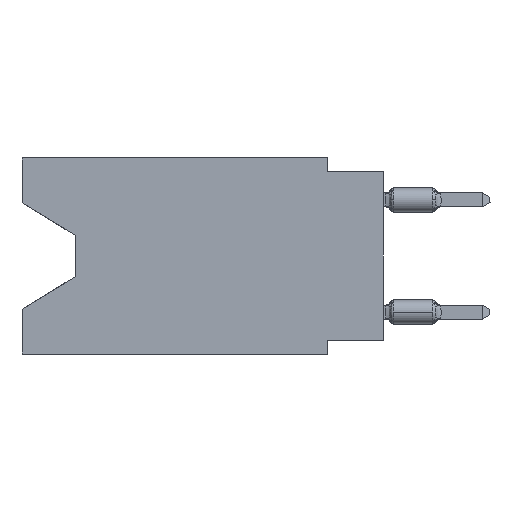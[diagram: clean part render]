
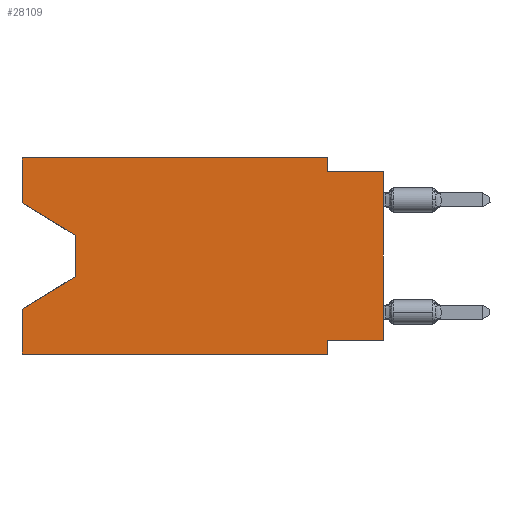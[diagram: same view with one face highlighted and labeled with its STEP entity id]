
A CAD part, left-side view. The second image highlights one B-rep face of the part: STEP entity #28109.
In plain terms, the highlighted planar face has unit normal (-1, 0, 0).
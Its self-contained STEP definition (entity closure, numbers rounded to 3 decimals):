
#141 = DIRECTION ( 'NONE',  ( 0., 0., 1. ) ) ;
#496 = EDGE_CURVE ( 'NONE', #2890, #24942, #21306, .T. ) ;
#534 = ORIENTED_EDGE ( 'NONE', *, *, #20708, .F. ) ;
#783 = CARTESIAN_POINT ( 'NONE',  ( 0., 2.54, 0. ) ) ;
#1128 = PLANE ( 'NONE',  #8096 ) ;
#2239 = LINE ( 'NONE', #45507, #47308 ) ;
#2470 = VECTOR ( 'NONE', #39328, 1000. ) ;
#2598 = CARTESIAN_POINT ( 'NONE',  ( 0., 16.383, -2.038 ) ) ;
#2780 = CARTESIAN_POINT ( 'NONE',  ( 0., 16.383, 0. ) ) ;
#2795 = CARTESIAN_POINT ( 'NONE',  ( 0., 13.97, -3.505 ) ) ;
#2890 = VERTEX_POINT ( 'NONE', #20108 ) ;
#3207 = ORIENTED_EDGE ( 'NONE', *, *, #7583, .F. ) ;
#3237 = CARTESIAN_POINT ( 'NONE',  ( 0., 2.54, -8.89 ) ) ;
#4053 = CARTESIAN_POINT ( 'NONE',  ( 0., 0., 0. ) ) ;
#4857 = EDGE_CURVE ( 'NONE', #46880, #24942, #29692, .T. ) ;
#7408 = CARTESIAN_POINT ( 'NONE',  ( 0., 0., -0.635 ) ) ;
#7494 = CARTESIAN_POINT ( 'NONE',  ( 0., 2.54, -0.635 ) ) ;
#7583 = EDGE_CURVE ( 'NONE', #36211, #30780, #2239, .T. ) ;
#7758 = CARTESIAN_POINT ( 'NONE',  ( 0., 13.97, -3.505 ) ) ;
#7838 = CARTESIAN_POINT ( 'NONE',  ( 0., 0., -0.635 ) ) ;
#8096 = AXIS2_PLACEMENT_3D ( 'NONE', #45171, #17316, #22001 ) ;
#9649 = ORIENTED_EDGE ( 'NONE', *, *, #20167, .F. ) ;
#9743 = CARTESIAN_POINT ( 'NONE',  ( 0., 2.54, -8.89 ) ) ;
#10964 = VECTOR ( 'NONE', #39224, 1000. ) ;
#11636 = VERTEX_POINT ( 'NONE', #2780 ) ;
#12014 = LINE ( 'NONE', #36253, #40355 ) ;
#12415 = VERTEX_POINT ( 'NONE', #2598 ) ;
#12582 = ORIENTED_EDGE ( 'NONE', *, *, #18851, .F. ) ;
#12710 = ORIENTED_EDGE ( 'NONE', *, *, #4857, .F. ) ;
#13790 = VERTEX_POINT ( 'NONE', #33418 ) ;
#14168 = CARTESIAN_POINT ( 'NONE',  ( 0., 0., -8.255 ) ) ;
#14323 = DIRECTION ( 'NONE',  ( 0., 0., 1. ) ) ;
#14593 = VERTEX_POINT ( 'NONE', #37706 ) ;
#14701 = VECTOR ( 'NONE', #38627, 1000. ) ;
#15559 = VECTOR ( 'NONE', #38350, 1000. ) ;
#16330 = LINE ( 'NONE', #4053, #36348 ) ;
#16443 = VECTOR ( 'NONE', #21216, 1000. ) ;
#17316 = DIRECTION ( 'NONE',  ( 1., 0., 0. ) ) ;
#17380 = EDGE_LOOP ( 'NONE', ( #46474, #43123, #34491, #12710, #20181, #534, #21304, #41673, #12582, #3207, #35628, #9649 ) ) ;
#17994 = VECTOR ( 'NONE', #26310, 1000. ) ;
#18348 = LINE ( 'NONE', #14168, #45370 ) ;
#18851 = EDGE_CURVE ( 'NONE', #30780, #36092, #23837, .T. ) ;
#20108 = CARTESIAN_POINT ( 'NONE',  ( 0., 13.97, -5.385 ) ) ;
#20167 = EDGE_CURVE ( 'NONE', #12415, #11636, #26368, .T. ) ;
#20181 = ORIENTED_EDGE ( 'NONE', *, *, #43624, .T. ) ;
#20708 = EDGE_CURVE ( 'NONE', #13790, #50838, #33207, .T. ) ;
#21216 = DIRECTION ( 'NONE',  ( 0., 0., -1. ) ) ;
#21304 = ORIENTED_EDGE ( 'NONE', *, *, #46533, .F. ) ;
#21306 = LINE ( 'NONE', #48915, #22105 ) ;
#22001 = DIRECTION ( 'NONE',  ( 0., 0., -1. ) ) ;
#22105 = VECTOR ( 'NONE', #49180, 1000. ) ;
#22454 = CARTESIAN_POINT ( 'NONE',  ( 0., 16.383, 0. ) ) ;
#23368 = EDGE_CURVE ( 'NONE', #32711, #2890, #31250, .T. ) ;
#23837 = LINE ( 'NONE', #7408, #10964 ) ;
#24278 = DIRECTION ( 'NONE',  ( 0., -1., 0. ) ) ;
#24942 = VERTEX_POINT ( 'NONE', #33313 ) ;
#26310 = DIRECTION ( 'NONE',  ( 0., -0.855, -0.519 ) ) ;
#26368 = LINE ( 'NONE', #22454, #15559 ) ;
#26617 = EDGE_CURVE ( 'NONE', #12415, #32711, #38030, .T. ) ;
#27095 = CARTESIAN_POINT ( 'NONE',  ( 0., 16.383, -8.89 ) ) ;
#28109 = ADVANCED_FACE ( 'NONE', ( #41293 ), #1128, .F. ) ;
#29427 = CARTESIAN_POINT ( 'NONE',  ( 0., 16.383, 0. ) ) ;
#29692 = LINE ( 'NONE', #29427, #41431 ) ;
#30780 = VERTEX_POINT ( 'NONE', #7494 ) ;
#31250 = LINE ( 'NONE', #7758, #2470 ) ;
#32711 = VERTEX_POINT ( 'NONE', #2795 ) ;
#33207 = LINE ( 'NONE', #9743, #16443 ) ;
#33313 = CARTESIAN_POINT ( 'NONE',  ( 0., 16.383, -6.852 ) ) ;
#33418 = CARTESIAN_POINT ( 'NONE',  ( 0., 2.54, -8.255 ) ) ;
#34491 = ORIENTED_EDGE ( 'NONE', *, *, #496, .T. ) ;
#35628 = ORIENTED_EDGE ( 'NONE', *, *, #38288, .F. ) ;
#36092 = VERTEX_POINT ( 'NONE', #7838 ) ;
#36211 = VERTEX_POINT ( 'NONE', #783 ) ;
#36253 = CARTESIAN_POINT ( 'NONE',  ( 0., 16.383, 0. ) ) ;
#36348 = VECTOR ( 'NONE', #141, 1000. ) ;
#37706 = CARTESIAN_POINT ( 'NONE',  ( 0., 0., -8.255 ) ) ;
#38030 = LINE ( 'NONE', #49999, #17994 ) ;
#38288 = EDGE_CURVE ( 'NONE', #11636, #36211, #12014, .T. ) ;
#38350 = DIRECTION ( 'NONE',  ( 0., 0., 1. ) ) ;
#38627 = DIRECTION ( 'NONE',  ( 0., -1., 0. ) ) ;
#38647 = DIRECTION ( 'NONE',  ( 0., 1., 0. ) ) ;
#39224 = DIRECTION ( 'NONE',  ( 0., -1., 0. ) ) ;
#39328 = DIRECTION ( 'NONE',  ( 0., 0., -1. ) ) ;
#40355 = VECTOR ( 'NONE', #24278, 1000. ) ;
#41293 = FACE_OUTER_BOUND ( 'NONE', #17380, .T. ) ;
#41431 = VECTOR ( 'NONE', #14323, 1000. ) ;
#41562 = EDGE_CURVE ( 'NONE', #14593, #36092, #16330, .T. ) ;
#41673 = ORIENTED_EDGE ( 'NONE', *, *, #41562, .T. ) ;
#42796 = LINE ( 'NONE', #46927, #14701 ) ;
#43123 = ORIENTED_EDGE ( 'NONE', *, *, #23368, .T. ) ;
#43624 = EDGE_CURVE ( 'NONE', #46880, #50838, #42796, .T. ) ;
#45171 = CARTESIAN_POINT ( 'NONE',  ( 0., 16.383, 0. ) ) ;
#45370 = VECTOR ( 'NONE', #38647, 1000. ) ;
#45507 = CARTESIAN_POINT ( 'NONE',  ( 0., 2.54, 0. ) ) ;
#46474 = ORIENTED_EDGE ( 'NONE', *, *, #26617, .T. ) ;
#46533 = EDGE_CURVE ( 'NONE', #14593, #13790, #18348, .T. ) ;
#46880 = VERTEX_POINT ( 'NONE', #27095 ) ;
#46927 = CARTESIAN_POINT ( 'NONE',  ( 0., 16.383, -8.89 ) ) ;
#47308 = VECTOR ( 'NONE', #49689, 1000. ) ;
#48915 = CARTESIAN_POINT ( 'NONE',  ( 0., 13.97, -5.385 ) ) ;
#49180 = DIRECTION ( 'NONE',  ( 0., 0.855, -0.519 ) ) ;
#49689 = DIRECTION ( 'NONE',  ( 0., 0., -1. ) ) ;
#49999 = CARTESIAN_POINT ( 'NONE',  ( 0., 16.383, -2.038 ) ) ;
#50838 = VERTEX_POINT ( 'NONE', #3237 ) ;
